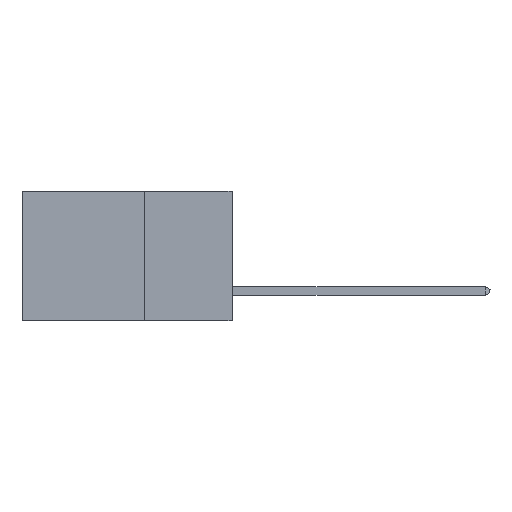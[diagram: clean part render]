
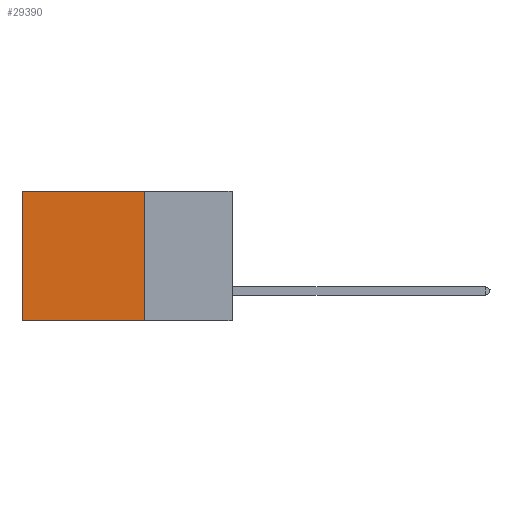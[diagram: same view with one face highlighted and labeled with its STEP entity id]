
A CAD part, left-side view. The second image highlights one B-rep face of the part: STEP entity #29390.
In plain terms, the highlighted planar face has unit normal (-1, 0, 0).
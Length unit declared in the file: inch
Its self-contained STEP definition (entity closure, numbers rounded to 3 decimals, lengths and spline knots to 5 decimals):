
#2961 = ORIENTED_EDGE ( 'NONE', *, *, #20677, .T. ) ;
#3313 = FACE_OUTER_BOUND ( 'NONE', #38413, .T. ) ;
#4010 = VECTOR ( 'NONE', #43608, 39.37008 ) ;
#5030 = VECTOR ( 'NONE', #34081, 39.37008 ) ;
#6028 = DIRECTION ( 'NONE',  ( 1., 0., 0. ) ) ;
#11447 = CARTESIAN_POINT ( 'NONE',  ( 0.2875, 0.25, 0. ) ) ;
#11548 = CARTESIAN_POINT ( 'NONE',  ( 0.2875, 0.25, -0.37 ) ) ;
#11939 = EDGE_CURVE ( 'NONE', #19333, #25285, #29708, .T. ) ;
#12076 = VECTOR ( 'NONE', #32747, 39.37008 ) ;
#13346 = CARTESIAN_POINT ( 'NONE',  ( 0.2875, 0.6, 0. ) ) ;
#16564 = LINE ( 'NONE', #11447, #12076 ) ;
#16772 = DIRECTION ( 'NONE',  ( 0., 0., -1. ) ) ;
#19333 = VERTEX_POINT ( 'NONE', #20845 ) ;
#20677 = EDGE_CURVE ( 'NONE', #40101, #43896, #32169, .T. ) ;
#20845 = CARTESIAN_POINT ( 'NONE',  ( 0.2875, 0.25, 0. ) ) ;
#21936 = VECTOR ( 'NONE', #24537, 39.37008 ) ;
#24082 = CARTESIAN_POINT ( 'NONE',  ( 0.2875, 0.25, 0. ) ) ;
#24537 = DIRECTION ( 'NONE',  ( 0., 0., -1. ) ) ;
#25285 = VERTEX_POINT ( 'NONE', #11548 ) ;
#25802 = CARTESIAN_POINT ( 'NONE',  ( 0.2875, 0.6, -0.37 ) ) ;
#25866 = CARTESIAN_POINT ( 'NONE',  ( 0.2875, 0.25, -0.37 ) ) ;
#27841 = CARTESIAN_POINT ( 'NONE',  ( 0.2875, 0.25, 0. ) ) ;
#29390 = ADVANCED_FACE ( 'NONE', ( #3313 ), #36840, .F. ) ;
#29708 = LINE ( 'NONE', #24082, #21936 ) ;
#32169 = LINE ( 'NONE', #43599, #5030 ) ;
#32747 = DIRECTION ( 'NONE',  ( 0., 1., 0. ) ) ;
#33549 = EDGE_CURVE ( 'NONE', #25285, #43896, #38914, .T. ) ;
#34081 = DIRECTION ( 'NONE',  ( 0., 0., -1. ) ) ;
#35353 = ORIENTED_EDGE ( 'NONE', *, *, #33549, .F. ) ;
#36521 = ORIENTED_EDGE ( 'NONE', *, *, #11939, .F. ) ;
#36840 = PLANE ( 'NONE',  #43030 ) ;
#38413 = EDGE_LOOP ( 'NONE', ( #2961, #35353, #36521, #42375 ) ) ;
#38914 = LINE ( 'NONE', #25866, #4010 ) ;
#40101 = VERTEX_POINT ( 'NONE', #13346 ) ;
#42008 = EDGE_CURVE ( 'NONE', #19333, #40101, #16564, .T. ) ;
#42375 = ORIENTED_EDGE ( 'NONE', *, *, #42008, .T. ) ;
#43030 = AXIS2_PLACEMENT_3D ( 'NONE', #27841, #6028, #16772 ) ;
#43599 = CARTESIAN_POINT ( 'NONE',  ( 0.2875, 0.6, 0. ) ) ;
#43608 = DIRECTION ( 'NONE',  ( 0., 1., 0. ) ) ;
#43896 = VERTEX_POINT ( 'NONE', #25802 ) ;
